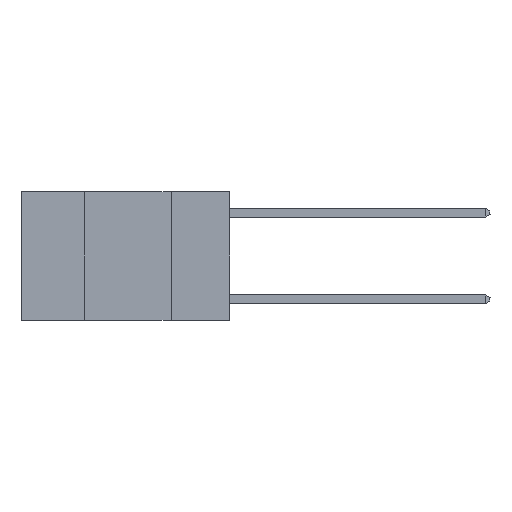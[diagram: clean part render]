
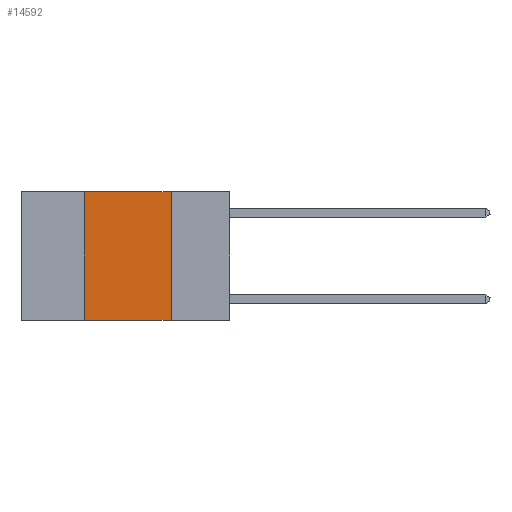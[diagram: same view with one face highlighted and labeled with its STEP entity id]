
A CAD part, left-side view. The second image highlights one B-rep face of the part: STEP entity #14592.
In plain terms, the highlighted planar face has unit normal (-1, 0, 0).
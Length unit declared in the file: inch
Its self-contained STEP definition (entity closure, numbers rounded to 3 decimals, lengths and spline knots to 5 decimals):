
#605 = CARTESIAN_POINT ( 'NONE',  ( 0., 0.42, 0. ) ) ;
#963 = VERTEX_POINT ( 'NONE', #3596 ) ;
#2355 = LINE ( 'NONE', #5127, #8782 ) ;
#2527 = EDGE_CURVE ( 'NONE', #8134, #6561, #4804, .T. ) ;
#3114 = VECTOR ( 'NONE', #5746, 39.37008 ) ;
#3596 = CARTESIAN_POINT ( 'NONE',  ( 0., 0.42, -0.37 ) ) ;
#4252 = ORIENTED_EDGE ( 'NONE', *, *, #5014, .F. ) ;
#4401 = LINE ( 'NONE', #605, #3114 ) ;
#4526 = DIRECTION ( 'NONE',  ( 0., 0., -1. ) ) ;
#4804 = LINE ( 'NONE', #13946, #5165 ) ;
#4914 = VERTEX_POINT ( 'NONE', #14466 ) ;
#5014 = EDGE_CURVE ( 'NONE', #4914, #8134, #2355, .T. ) ;
#5127 = CARTESIAN_POINT ( 'NONE',  ( 0., 0.6, 0. ) ) ;
#5165 = VECTOR ( 'NONE', #15038, 39.37008 ) ;
#5194 = EDGE_LOOP ( 'NONE', ( #16194, #4252, #12165, #13050 ) ) ;
#5746 = DIRECTION ( 'NONE',  ( 0., 0., 1. ) ) ;
#5773 = CARTESIAN_POINT ( 'NONE',  ( 0., 0.17, 0. ) ) ;
#5843 = CARTESIAN_POINT ( 'NONE',  ( 0., 0.6, -0.37 ) ) ;
#6111 = DIRECTION ( 'NONE',  ( 1., 0., 0. ) ) ;
#6329 = VECTOR ( 'NONE', #9776, 39.37008 ) ;
#6561 = VERTEX_POINT ( 'NONE', #13137 ) ;
#7136 = EDGE_CURVE ( 'NONE', #963, #6561, #16268, .T. ) ;
#7298 = CARTESIAN_POINT ( 'NONE',  ( 0., 0.6, 0. ) ) ;
#8134 = VERTEX_POINT ( 'NONE', #5773 ) ;
#8782 = VECTOR ( 'NONE', #15104, 39.37008 ) ;
#9714 = PLANE ( 'NONE',  #14935 ) ;
#9776 = DIRECTION ( 'NONE',  ( 0., -1., 0. ) ) ;
#12165 = ORIENTED_EDGE ( 'NONE', *, *, #12311, .F. ) ;
#12234 = FACE_OUTER_BOUND ( 'NONE', #5194, .T. ) ;
#12311 = EDGE_CURVE ( 'NONE', #963, #4914, #4401, .T. ) ;
#13050 = ORIENTED_EDGE ( 'NONE', *, *, #7136, .T. ) ;
#13137 = CARTESIAN_POINT ( 'NONE',  ( 0., 0.17, -0.37 ) ) ;
#13946 = CARTESIAN_POINT ( 'NONE',  ( 0., 0.17, 0. ) ) ;
#14466 = CARTESIAN_POINT ( 'NONE',  ( 0., 0.42, 0. ) ) ;
#14592 = ADVANCED_FACE ( 'NONE', ( #12234 ), #9714, .F. ) ;
#14935 = AXIS2_PLACEMENT_3D ( 'NONE', #7298, #6111, #4526 ) ;
#15038 = DIRECTION ( 'NONE',  ( 0., 0., -1. ) ) ;
#15104 = DIRECTION ( 'NONE',  ( 0., -1., 0. ) ) ;
#16194 = ORIENTED_EDGE ( 'NONE', *, *, #2527, .F. ) ;
#16268 = LINE ( 'NONE', #5843, #6329 ) ;
